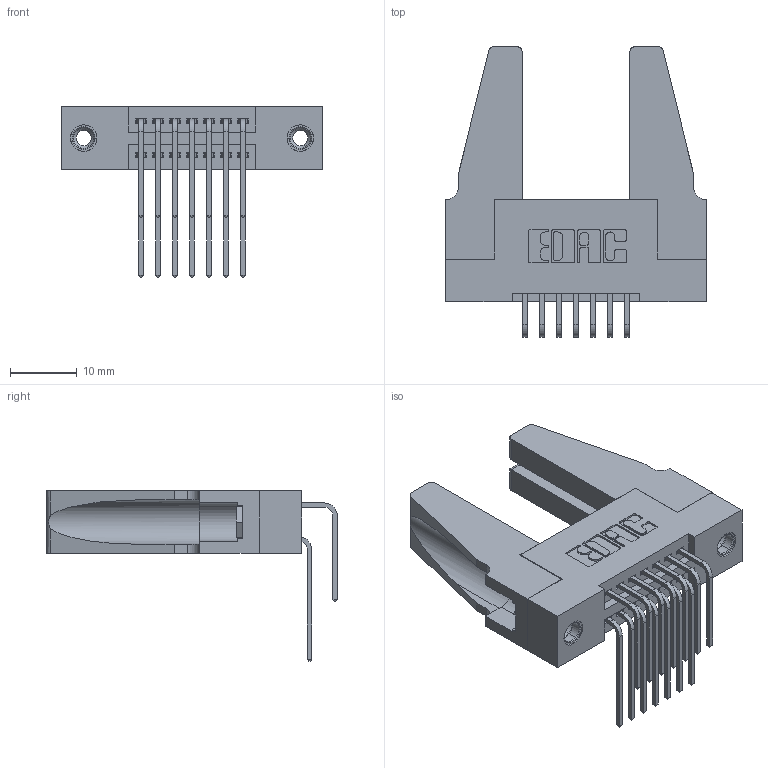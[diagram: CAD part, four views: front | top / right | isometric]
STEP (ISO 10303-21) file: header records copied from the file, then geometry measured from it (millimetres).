
FILE_DESCRIPTION (( 'STEP AP203' ), '1' );
FILE_NAME ('345-014-559-288.STEP', '2019-10-26T19:25:02', ( '' ), ( '' ), 'SwSTEP 2.0', 'SolidWorks 2016', '' );
FILE_SCHEMA (( 'CONFIG_CONTROL_DESIGN' ));
Length unit declared in the file: inch
Products named in the file (6): 345-292-001_559 Tail - 2; 345-220-078_345-220-088; 345 Part_Flush Mounting Lugs - 0.156 Dia-TH; 345-292-001_558 559 Tail - 1; 345-250-001_345-250-001-102; 345-014-559-288
Assembly tree (19 placements, depth 2):
  345-014-559-288
    345 Part_Flush Mounting Lugs - 0.156 Dia-TH
    345-292-001_558 559 Tail - 1  x7
    345-292-001_559 Tail - 2  x7
    345-250-001_345-250-001-102  x2
    345-220-078_345-220-088  x2
Bounding box: 39.01 x 43.42 x 25.53 mm (x, y, z)
Volume: 6798.2 mm3; surface area: 8065.3 mm2
Topology: 19 solids, 19 shells, 978 faces, 2825 edges, 1854 vertices
Faces by surface type: plane 642, cylinder 320, cone 12, torus 4
Entity records: 14004 total; most frequent: CARTESIAN_POINT 2421, ORIENTED_EDGE 2264, DIRECTION 2156, EDGE_CURVE 1132, LINE 890, VECTOR 890, VERTEX_POINT 746, AXIS2_PLACEMENT_3D 633
